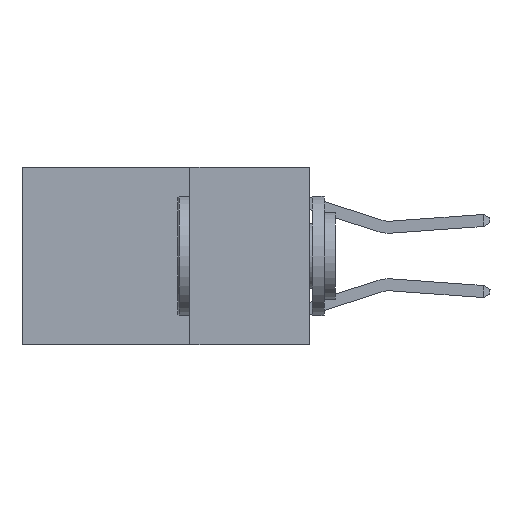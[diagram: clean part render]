
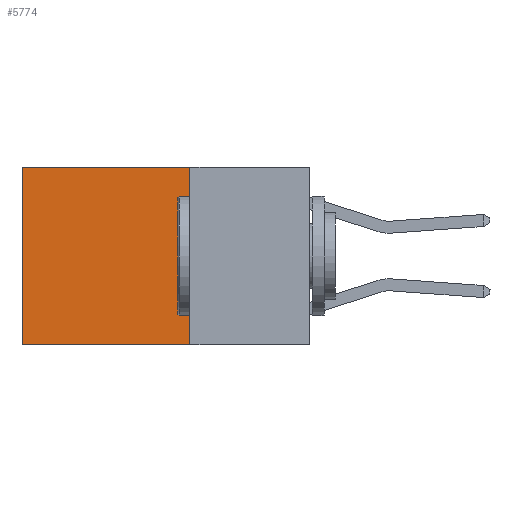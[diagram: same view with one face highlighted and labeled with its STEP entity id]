
A CAD part, left-side view. The second image highlights one B-rep face of the part: STEP entity #5774.
In plain terms, the highlighted planar face has unit normal (-1, 0, 0).
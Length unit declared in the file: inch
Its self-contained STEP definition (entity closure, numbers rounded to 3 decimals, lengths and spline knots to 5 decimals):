
#363 = VECTOR ( 'NONE', #12996, 39.37008 ) ;
#2120 = EDGE_CURVE ( 'NONE', #5629, #6270, #10760, .T. ) ;
#2873 = CARTESIAN_POINT ( 'NONE',  ( 0.2625, 0.6, 0. ) ) ;
#3418 = EDGE_LOOP ( 'NONE', ( #19546, #22165, #12519, #17492 ) ) ;
#3675 = DIRECTION ( 'NONE',  ( 0., 0., -1. ) ) ;
#3709 = CARTESIAN_POINT ( 'NONE',  ( 0.2625, 0.25, -0.37 ) ) ;
#4505 = EDGE_CURVE ( 'NONE', #7511, #18088, #16476, .T. ) ;
#5629 = VERTEX_POINT ( 'NONE', #20030 ) ;
#5774 = ADVANCED_FACE ( 'NONE', ( #26606 ), #24667, .F. ) ;
#5864 = CARTESIAN_POINT ( 'NONE',  ( 0.2625, 0.25, 0. ) ) ;
#6270 = VERTEX_POINT ( 'NONE', #10399 ) ;
#7511 = VERTEX_POINT ( 'NONE', #3709 ) ;
#7715 = CARTESIAN_POINT ( 'NONE',  ( 0.2625, 0.25, 0. ) ) ;
#7988 = DIRECTION ( 'NONE',  ( 0., 0., -1. ) ) ;
#9336 = VECTOR ( 'NONE', #3675, 39.37008 ) ;
#10399 = CARTESIAN_POINT ( 'NONE',  ( 0.2625, 0.6, 0. ) ) ;
#10760 = LINE ( 'NONE', #11035, #23647 ) ;
#11035 = CARTESIAN_POINT ( 'NONE',  ( 0.2625, 0.25, 0. ) ) ;
#12519 = ORIENTED_EDGE ( 'NONE', *, *, #13618, .F. ) ;
#12996 = DIRECTION ( 'NONE',  ( 0., 0., -1. ) ) ;
#13618 = EDGE_CURVE ( 'NONE', #5629, #7511, #20509, .T. ) ;
#13865 = DIRECTION ( 'NONE',  ( 1., 0., 0. ) ) ;
#16476 = LINE ( 'NONE', #25074, #23323 ) ;
#17251 = CARTESIAN_POINT ( 'NONE',  ( 0.2625, 0.6, -0.37 ) ) ;
#17492 = ORIENTED_EDGE ( 'NONE', *, *, #2120, .T. ) ;
#18088 = VERTEX_POINT ( 'NONE', #17251 ) ;
#19122 = DIRECTION ( 'NONE',  ( 0., 1., 0. ) ) ;
#19546 = ORIENTED_EDGE ( 'NONE', *, *, #23774, .T. ) ;
#20030 = CARTESIAN_POINT ( 'NONE',  ( 0.2625, 0.25, 0. ) ) ;
#20509 = LINE ( 'NONE', #5864, #9336 ) ;
#22165 = ORIENTED_EDGE ( 'NONE', *, *, #4505, .F. ) ;
#23323 = VECTOR ( 'NONE', #24950, 39.37008 ) ;
#23408 = LINE ( 'NONE', #2873, #363 ) ;
#23647 = VECTOR ( 'NONE', #19122, 39.37008 ) ;
#23774 = EDGE_CURVE ( 'NONE', #6270, #18088, #23408, .T. ) ;
#23985 = AXIS2_PLACEMENT_3D ( 'NONE', #7715, #13865, #7988 ) ;
#24667 = PLANE ( 'NONE',  #23985 ) ;
#24950 = DIRECTION ( 'NONE',  ( 0., 1., 0. ) ) ;
#25074 = CARTESIAN_POINT ( 'NONE',  ( 0.2625, 0.25, -0.37 ) ) ;
#26606 = FACE_OUTER_BOUND ( 'NONE', #3418, .T. ) ;
